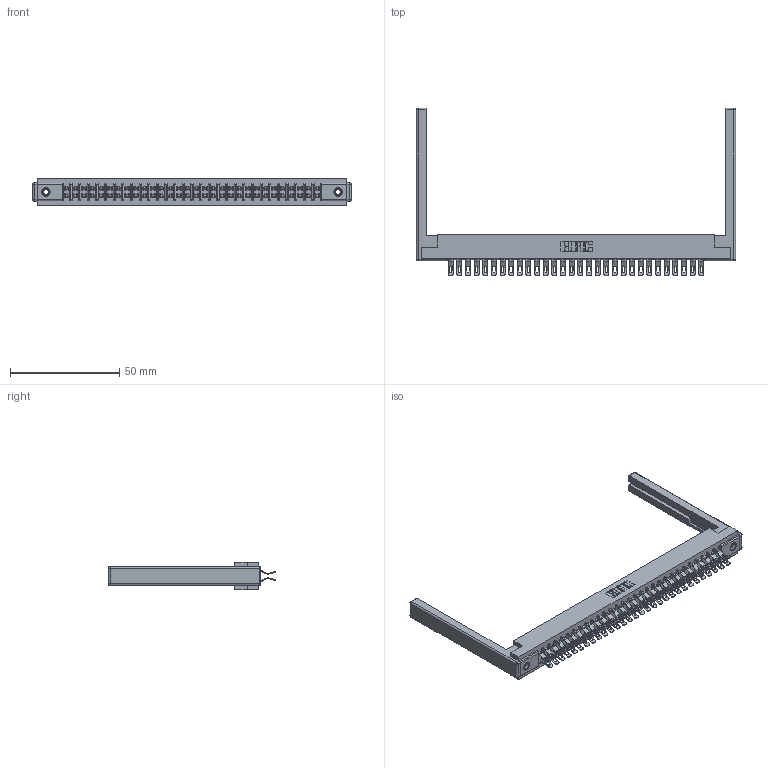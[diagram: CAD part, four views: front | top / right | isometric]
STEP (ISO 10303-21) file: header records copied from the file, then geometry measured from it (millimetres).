
FILE_DESCRIPTION (( 'STEP AP203' ), '1' );
FILE_NAME ('307-060-455-268.STEP', '2020-09-30T15:06:32', ( '' ), ( '' ), 'SwSTEP 2.0', 'SolidWorks 2020', '' );
FILE_SCHEMA (( 'CONFIG_CONTROL_DESIGN' ));
Length unit declared in the file: inch
Products named in the file (5): 307 Part_.156 Dia Mounting Holes; 307-290-001_555; 307-060-455-268; 345-250-001_345-250-001-102; 307-220-068
Assembly tree (65 placements, depth 2):
  307-060-455-268
    307 Part_.156 Dia Mounting Holes
    307-290-001_555  x60
    307-220-068  x2
    345-250-001_345-250-001-102  x2
Bounding box: 146.3 x 76.71 x 12.7 mm (x, y, z)
Volume: 20032 mm3; surface area: 23882.4 mm2
Topology: 65 solids, 65 shells, 3963 faces, 11573 edges, 7530 vertices
Faces by surface type: plane 2198, cylinder 1679, sphere 70, cone 12, torus 4
Entity records: 31454 total; most frequent: CARTESIAN_POINT 5131, ORIENTED_EDGE 5078, DIRECTION 5053, EDGE_CURVE 2539, VECTOR 1929, LINE 1929, VERTEX_POINT 1640, AXIS2_PLACEMENT_3D 1562
